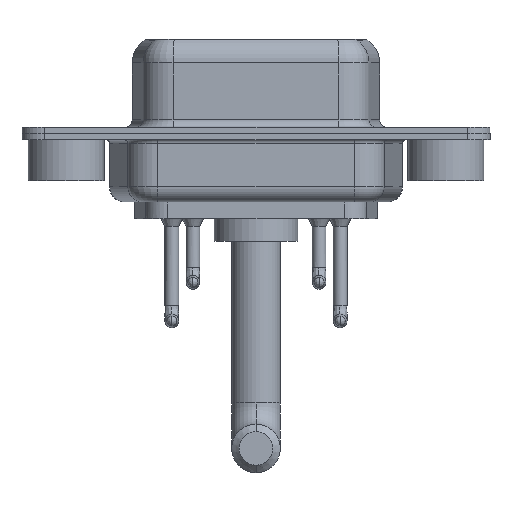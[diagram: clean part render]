
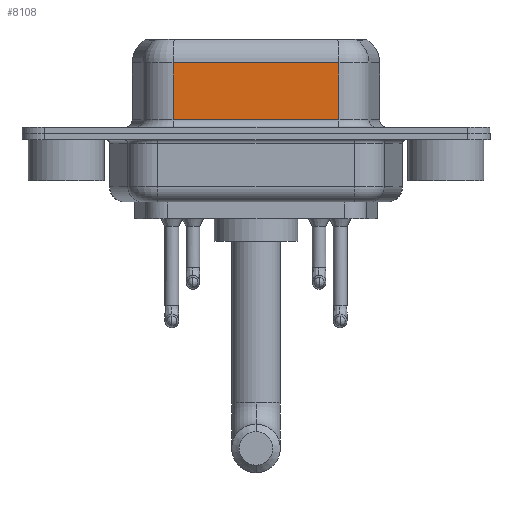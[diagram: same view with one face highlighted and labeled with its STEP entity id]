
A CAD part, front view. The second image highlights one B-rep face of the part: STEP entity #8108.
In plain terms, the highlighted planar face has unit normal (0, -1, 0).
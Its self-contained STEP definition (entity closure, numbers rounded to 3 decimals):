
#633 = VECTOR ( 'NONE', #16241, 1000. ) ;
#1344 = DIRECTION ( 'NONE',  ( -1., 0., 0. ) ) ;
#1555 = VERTEX_POINT ( 'NONE', #2878 ) ;
#2351 = EDGE_CURVE ( 'NONE', #12080, #1555, #15697, .T. ) ;
#2409 = PLANE ( 'NONE',  #14440 ) ;
#2608 = LINE ( 'NONE', #10051, #4710 ) ;
#2789 = VECTOR ( 'NONE', #8379, 1000. ) ;
#2878 = CARTESIAN_POINT ( 'NONE',  ( 7.038, -3.95, 0.9 ) ) ;
#3575 = DIRECTION ( 'NONE',  ( 0., 1., 0. ) ) ;
#4299 = CARTESIAN_POINT ( 'NONE',  ( 17.962, -3.95, 0.9 ) ) ;
#4302 = EDGE_CURVE ( 'NONE', #8278, #5125, #9918, .T. ) ;
#4710 = VECTOR ( 'NONE', #8985, 1000. ) ;
#5125 = VERTEX_POINT ( 'NONE', #4299 ) ;
#5584 = LINE ( 'NONE', #14232, #15457 ) ;
#7621 = FACE_OUTER_BOUND ( 'NONE', #14825, .T. ) ;
#7948 = CARTESIAN_POINT ( 'NONE',  ( 17.962, -3.95, 4.65 ) ) ;
#8005 = ORIENTED_EDGE ( 'NONE', *, *, #4302, .F. ) ;
#8108 = ADVANCED_FACE ( 'NONE', ( #7621 ), #2409, .F. ) ;
#8278 = VERTEX_POINT ( 'NONE', #7948 ) ;
#8303 = DIRECTION ( 'NONE',  ( -1., 0., 0. ) ) ;
#8379 = DIRECTION ( 'NONE',  ( 0., 0., -1. ) ) ;
#8985 = DIRECTION ( 'NONE',  ( 1., 0., 0. ) ) ;
#9039 = ORIENTED_EDGE ( 'NONE', *, *, #11131, .T. ) ;
#9918 = LINE ( 'NONE', #11222, #633 ) ;
#10051 = CARTESIAN_POINT ( 'NONE',  ( 17.962, -3.95, 0.9 ) ) ;
#11131 = EDGE_CURVE ( 'NONE', #8278, #12080, #5584, .T. ) ;
#11222 = CARTESIAN_POINT ( 'NONE',  ( 17.962, -3.95, 6.4 ) ) ;
#12080 = VERTEX_POINT ( 'NONE', #14766 ) ;
#12365 = ORIENTED_EDGE ( 'NONE', *, *, #2351, .T. ) ;
#12635 = CARTESIAN_POINT ( 'NONE',  ( 17.962, -3.95, 6.4 ) ) ;
#14232 = CARTESIAN_POINT ( 'NONE',  ( 17.962, -3.95, 4.65 ) ) ;
#14440 = AXIS2_PLACEMENT_3D ( 'NONE', #12635, #3575, #1344 ) ;
#14766 = CARTESIAN_POINT ( 'NONE',  ( 7.038, -3.95, 4.65 ) ) ;
#14825 = EDGE_LOOP ( 'NONE', ( #8005, #9039, #12365, #15133 ) ) ;
#15133 = ORIENTED_EDGE ( 'NONE', *, *, #15416, .T. ) ;
#15416 = EDGE_CURVE ( 'NONE', #1555, #5125, #2608, .T. ) ;
#15457 = VECTOR ( 'NONE', #8303, 1000. ) ;
#15697 = LINE ( 'NONE', #16022, #2789 ) ;
#16022 = CARTESIAN_POINT ( 'NONE',  ( 7.038, -3.95, 6.4 ) ) ;
#16241 = DIRECTION ( 'NONE',  ( 0., 0., -1. ) ) ;
